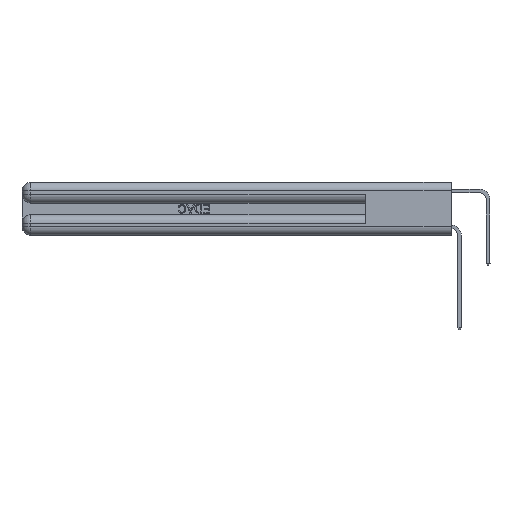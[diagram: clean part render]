
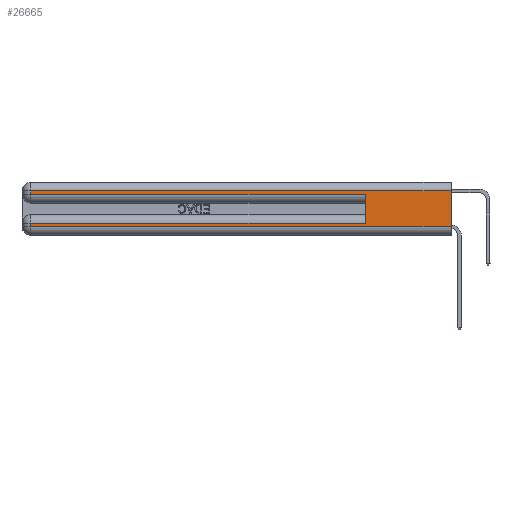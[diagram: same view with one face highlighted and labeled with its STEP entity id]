
A CAD part, left-side view. The second image highlights one B-rep face of the part: STEP entity #26665.
In plain terms, the highlighted planar face has unit normal (-1, 0, 0).
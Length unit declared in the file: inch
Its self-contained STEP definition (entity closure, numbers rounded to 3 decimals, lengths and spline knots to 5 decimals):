
#259 = EDGE_CURVE ( 'NONE', #19481, #27094, #6638, .T. ) ;
#354 = CARTESIAN_POINT ( 'NONE',  ( 0., 0., 0.31 ) ) ;
#607 = DIRECTION ( 'NONE',  ( 0., -1., 0. ) ) ;
#862 = CARTESIAN_POINT ( 'NONE',  ( 0., 0., 0.37 ) ) ;
#2107 = EDGE_CURVE ( 'NONE', #22248, #27403, #18955, .T. ) ;
#2971 = EDGE_CURVE ( 'NONE', #27403, #4685, #6509, .T. ) ;
#3210 = EDGE_CURVE ( 'NONE', #19481, #22248, #15668, .T. ) ;
#3314 = VECTOR ( 'NONE', #26624, 39.37008 ) ;
#4562 = VERTEX_POINT ( 'NONE', #11254 ) ;
#4685 = VERTEX_POINT ( 'NONE', #16472 ) ;
#4716 = CARTESIAN_POINT ( 'NONE',  ( 0., 0., 0.06 ) ) ;
#5193 = VECTOR ( 'NONE', #13271, 39.37008 ) ;
#5230 = ORIENTED_EDGE ( 'NONE', *, *, #2107, .T. ) ;
#5444 = LINE ( 'NONE', #19716, #3314 ) ;
#5689 = CARTESIAN_POINT ( 'NONE',  ( 0., 0., 0.285 ) ) ;
#5717 = VECTOR ( 'NONE', #26377, 39.37008 ) ;
#6509 = LINE ( 'NONE', #5689, #12272 ) ;
#6638 = LINE ( 'NONE', #27180, #5193 ) ;
#6949 = ORIENTED_EDGE ( 'NONE', *, *, #2971, .T. ) ;
#6955 = ORIENTED_EDGE ( 'NONE', *, *, #23681, .F. ) ;
#7013 = LINE ( 'NONE', #14862, #29309 ) ;
#7326 = CARTESIAN_POINT ( 'NONE',  ( 0., 0., 0.06 ) ) ;
#7365 = VERTEX_POINT ( 'NONE', #26268 ) ;
#7482 = DIRECTION ( 'NONE',  ( 0., 0., -1. ) ) ;
#7698 = FACE_OUTER_BOUND ( 'NONE', #14642, .T. ) ;
#7930 = EDGE_CURVE ( 'NONE', #4562, #27094, #13266, .T. ) ;
#9975 = DIRECTION ( 'NONE',  ( 1., 0., 0. ) ) ;
#11254 = CARTESIAN_POINT ( 'NONE',  ( 0., 2.94, 0.06 ) ) ;
#12272 = VECTOR ( 'NONE', #26255, 39.37008 ) ;
#12348 = CARTESIAN_POINT ( 'NONE',  ( 0., 0.6, 0.145 ) ) ;
#12617 = CARTESIAN_POINT ( 'NONE',  ( 0., 0.6, 0.085 ) ) ;
#13266 = LINE ( 'NONE', #4716, #24885 ) ;
#13271 = DIRECTION ( 'NONE',  ( 0., 0., -1. ) ) ;
#13479 = VECTOR ( 'NONE', #29030, 39.37008 ) ;
#14642 = EDGE_LOOP ( 'NONE', ( #28493, #21297, #5230, #6949, #6955, #27140, #21548, #25265 ) ) ;
#14862 = CARTESIAN_POINT ( 'NONE',  ( 0., 2.94, 0.37 ) ) ;
#14889 = EDGE_CURVE ( 'NONE', #7365, #4562, #7013, .T. ) ;
#15668 = LINE ( 'NONE', #20470, #20041 ) ;
#15706 = AXIS2_PLACEMENT_3D ( 'NONE', #862, #9975, #28387 ) ;
#16472 = CARTESIAN_POINT ( 'NONE',  ( 0., 0.6, 0.285 ) ) ;
#17812 = EDGE_CURVE ( 'NONE', #26621, #7365, #5444, .T. ) ;
#18955 = LINE ( 'NONE', #26483, #13479 ) ;
#19481 = VERTEX_POINT ( 'NONE', #354 ) ;
#19716 = CARTESIAN_POINT ( 'NONE',  ( 0., 0., 0.085 ) ) ;
#20041 = VECTOR ( 'NONE', #27147, 39.37008 ) ;
#20470 = CARTESIAN_POINT ( 'NONE',  ( 0., 0., 0.31 ) ) ;
#20783 = CARTESIAN_POINT ( 'NONE',  ( 0., 2.94, 0.31 ) ) ;
#21297 = ORIENTED_EDGE ( 'NONE', *, *, #3210, .T. ) ;
#21548 = ORIENTED_EDGE ( 'NONE', *, *, #14889, .T. ) ;
#22248 = VERTEX_POINT ( 'NONE', #20783 ) ;
#22440 = CARTESIAN_POINT ( 'NONE',  ( 0., 2.94, 0.285 ) ) ;
#23681 = EDGE_CURVE ( 'NONE', #26621, #4685, #29115, .T. ) ;
#24885 = VECTOR ( 'NONE', #607, 39.37008 ) ;
#25265 = ORIENTED_EDGE ( 'NONE', *, *, #7930, .T. ) ;
#26255 = DIRECTION ( 'NONE',  ( 0., -1., 0. ) ) ;
#26268 = CARTESIAN_POINT ( 'NONE',  ( 0., 2.94, 0.085 ) ) ;
#26377 = DIRECTION ( 'NONE',  ( 0., 0., 1. ) ) ;
#26483 = CARTESIAN_POINT ( 'NONE',  ( 0., 2.94, 0.37 ) ) ;
#26621 = VERTEX_POINT ( 'NONE', #12617 ) ;
#26624 = DIRECTION ( 'NONE',  ( 0., 1., 0. ) ) ;
#26665 = ADVANCED_FACE ( 'NONE', ( #7698 ), #28801, .F. ) ;
#27094 = VERTEX_POINT ( 'NONE', #7326 ) ;
#27140 = ORIENTED_EDGE ( 'NONE', *, *, #17812, .T. ) ;
#27147 = DIRECTION ( 'NONE',  ( 0., 1., 0. ) ) ;
#27180 = CARTESIAN_POINT ( 'NONE',  ( 0., 0., 0.37 ) ) ;
#27403 = VERTEX_POINT ( 'NONE', #22440 ) ;
#28387 = DIRECTION ( 'NONE',  ( 0., 0., -1. ) ) ;
#28493 = ORIENTED_EDGE ( 'NONE', *, *, #259, .F. ) ;
#28801 = PLANE ( 'NONE',  #15706 ) ;
#29030 = DIRECTION ( 'NONE',  ( 0., 0., -1. ) ) ;
#29115 = LINE ( 'NONE', #12348, #5717 ) ;
#29309 = VECTOR ( 'NONE', #7482, 39.37008 ) ;
